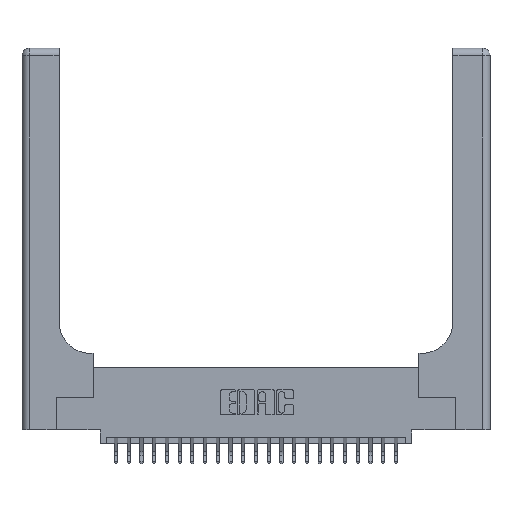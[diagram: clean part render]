
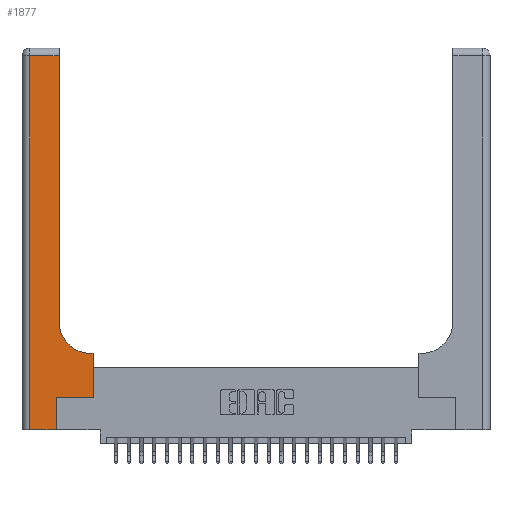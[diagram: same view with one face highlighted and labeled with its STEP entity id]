
A CAD part, top view. The second image highlights one B-rep face of the part: STEP entity #1877.
In plain terms, the highlighted planar face has unit normal (0, 0, 1).
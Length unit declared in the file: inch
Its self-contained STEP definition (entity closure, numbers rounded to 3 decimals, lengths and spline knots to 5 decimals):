
#35 = CARTESIAN_POINT ( 'NONE',  ( 0., 0., 0.37 ) ) ;
#159 = CARTESIAN_POINT ( 'NONE',  ( 0.5415, 0.85, 0.37 ) ) ;
#205 = VECTOR ( 'NONE', #23191, 39.37008 ) ;
#520 = DIRECTION ( 'NONE',  ( 0., 1., 0. ) ) ;
#637 = EDGE_CURVE ( 'NONE', #4243, #4184, #20480, .T. ) ;
#645 = CARTESIAN_POINT ( 'NONE',  ( 0., 2.94, 0.37 ) ) ;
#976 = VERTEX_POINT ( 'NONE', #1855 ) ;
#1480 = EDGE_CURVE ( 'NONE', #976, #8037, #10670, .T. ) ;
#1573 = VERTEX_POINT ( 'NONE', #6604 ) ;
#1855 = CARTESIAN_POINT ( 'NONE',  ( 0.5585, 0.25, 0.37 ) ) ;
#1877 = ADVANCED_FACE ( 'NONE', ( #20543 ), #14783, .F. ) ;
#2015 = CARTESIAN_POINT ( 'NONE',  ( 0.06, 2.94, 0.37 ) ) ;
#2234 = CARTESIAN_POINT ( 'NONE',  ( 0.5585, 0.25, 0.37 ) ) ;
#2334 = EDGE_CURVE ( 'NONE', #5184, #976, #3185, .T. ) ;
#2513 = VECTOR ( 'NONE', #8115, 39.37008 ) ;
#2544 = DIRECTION ( 'NONE',  ( -1., 0., 0. ) ) ;
#2560 = CARTESIAN_POINT ( 'NONE',  ( 0.06, 0., 0.37 ) ) ;
#2562 = DIRECTION ( 'NONE',  ( -1., 0., 0. ) ) ;
#2619 = CARTESIAN_POINT ( 'NONE',  ( 0.269, 0., 0.37 ) ) ;
#2759 = DIRECTION ( 'NONE',  ( 0., 1., 0. ) ) ;
#2996 = ORIENTED_EDGE ( 'NONE', *, *, #5394, .T. ) ;
#3185 = LINE ( 'NONE', #13589, #2513 ) ;
#4184 = VERTEX_POINT ( 'NONE', #23796 ) ;
#4239 = ORIENTED_EDGE ( 'NONE', *, *, #10282, .T. ) ;
#4243 = VERTEX_POINT ( 'NONE', #2560 ) ;
#4658 = CARTESIAN_POINT ( 'NONE',  ( 0.2915, 0.85, 0.37 ) ) ;
#4783 = CARTESIAN_POINT ( 'NONE',  ( 0.2915, 0.6, 0.37 ) ) ;
#5184 = VERTEX_POINT ( 'NONE', #17428 ) ;
#5194 = LINE ( 'NONE', #21170, #205 ) ;
#5394 = EDGE_CURVE ( 'NONE', #8037, #23240, #8339, .T. ) ;
#5472 = CIRCLE ( 'NONE', #20324, 0.25 ) ;
#5738 = EDGE_CURVE ( 'NONE', #23240, #13734, #5472, .T. ) ;
#6290 = ORIENTED_EDGE ( 'NONE', *, *, #1480, .T. ) ;
#6384 = VERTEX_POINT ( 'NONE', #2015 ) ;
#6435 = VECTOR ( 'NONE', #15027, 39.37008 ) ;
#6537 = CARTESIAN_POINT ( 'NONE',  ( 0.06, 3., 0.37 ) ) ;
#6604 = CARTESIAN_POINT ( 'NONE',  ( 0.2915, 2.94, 0.37 ) ) ;
#6631 = EDGE_LOOP ( 'NONE', ( #20141, #21697, #4239, #24173, #19342, #22623, #6290, #2996, #20919 ) ) ;
#8037 = VERTEX_POINT ( 'NONE', #19546 ) ;
#8115 = DIRECTION ( 'NONE',  ( 1., 0., 0. ) ) ;
#8339 = LINE ( 'NONE', #4783, #6435 ) ;
#10282 = EDGE_CURVE ( 'NONE', #6384, #4243, #24700, .T. ) ;
#10568 = DIRECTION ( 'NONE',  ( 0., 0., -1. ) ) ;
#10670 = LINE ( 'NONE', #2234, #14111 ) ;
#11012 = VECTOR ( 'NONE', #2562, 39.37008 ) ;
#11322 = AXIS2_PLACEMENT_3D ( 'NONE', #14503, #10568, #2544 ) ;
#12239 = VECTOR ( 'NONE', #16244, 39.37008 ) ;
#13589 = CARTESIAN_POINT ( 'NONE',  ( 0.269, 0.25, 0.37 ) ) ;
#13655 = VECTOR ( 'NONE', #520, 39.37008 ) ;
#13734 = VERTEX_POINT ( 'NONE', #4658 ) ;
#14111 = VECTOR ( 'NONE', #2759, 39.37008 ) ;
#14209 = VECTOR ( 'NONE', #16384, 39.37008 ) ;
#14503 = CARTESIAN_POINT ( 'NONE',  ( 0., 3., 0.37 ) ) ;
#14783 = PLANE ( 'NONE',  #11322 ) ;
#15027 = DIRECTION ( 'NONE',  ( -1., 0., 0. ) ) ;
#16244 = DIRECTION ( 'NONE',  ( 1., 0., 0. ) ) ;
#16265 = DIRECTION ( 'NONE',  ( 0., 0., -1. ) ) ;
#16384 = DIRECTION ( 'NONE',  ( 0., -1., 0. ) ) ;
#16534 = EDGE_CURVE ( 'NONE', #13734, #1573, #5194, .T. ) ;
#17428 = CARTESIAN_POINT ( 'NONE',  ( 0.269, 0.25, 0.37 ) ) ;
#18336 = DIRECTION ( 'NONE',  ( 1., 0., 0. ) ) ;
#19342 = ORIENTED_EDGE ( 'NONE', *, *, #21840, .T. ) ;
#19546 = CARTESIAN_POINT ( 'NONE',  ( 0.5585, 0.6, 0.37 ) ) ;
#19853 = LINE ( 'NONE', #645, #11012 ) ;
#20141 = ORIENTED_EDGE ( 'NONE', *, *, #16534, .T. ) ;
#20324 = AXIS2_PLACEMENT_3D ( 'NONE', #159, #16265, #18336 ) ;
#20480 = LINE ( 'NONE', #35, #12239 ) ;
#20543 = FACE_OUTER_BOUND ( 'NONE', #6631, .T. ) ;
#20919 = ORIENTED_EDGE ( 'NONE', *, *, #5738, .T. ) ;
#20980 = EDGE_CURVE ( 'NONE', #1573, #6384, #19853, .T. ) ;
#21170 = CARTESIAN_POINT ( 'NONE',  ( 0.2915, 3., 0.37 ) ) ;
#21697 = ORIENTED_EDGE ( 'NONE', *, *, #20980, .T. ) ;
#21840 = EDGE_CURVE ( 'NONE', #4184, #5184, #24454, .T. ) ;
#22029 = CARTESIAN_POINT ( 'NONE',  ( 0.5415, 0.6, 0.37 ) ) ;
#22623 = ORIENTED_EDGE ( 'NONE', *, *, #2334, .T. ) ;
#23191 = DIRECTION ( 'NONE',  ( 0., 1., 0. ) ) ;
#23240 = VERTEX_POINT ( 'NONE', #22029 ) ;
#23796 = CARTESIAN_POINT ( 'NONE',  ( 0.269, 0., 0.37 ) ) ;
#24173 = ORIENTED_EDGE ( 'NONE', *, *, #637, .T. ) ;
#24454 = LINE ( 'NONE', #2619, #13655 ) ;
#24700 = LINE ( 'NONE', #6537, #14209 ) ;
